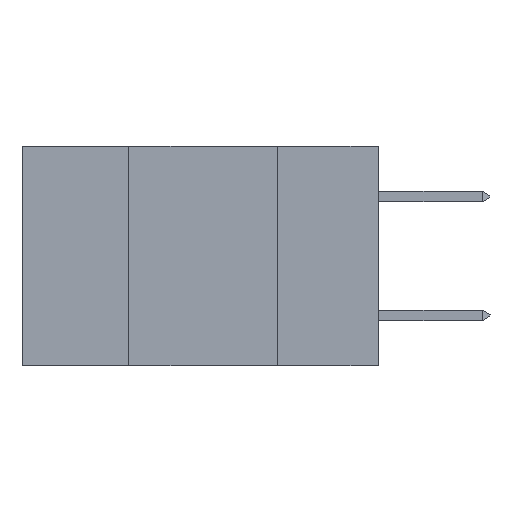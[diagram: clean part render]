
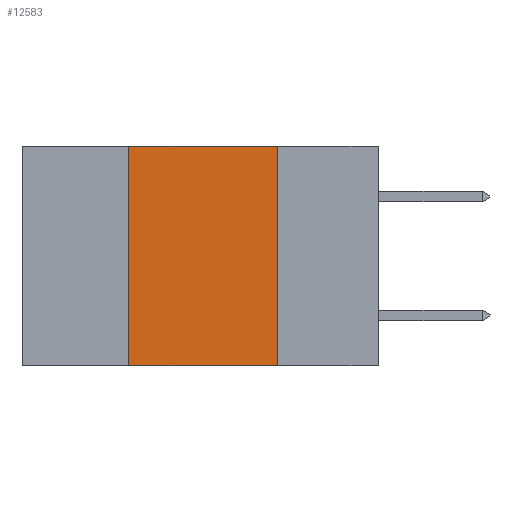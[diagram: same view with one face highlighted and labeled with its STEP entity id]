
A CAD part, left-side view. The second image highlights one B-rep face of the part: STEP entity #12583.
In plain terms, the highlighted planar face has unit normal (-1, 0, 0).
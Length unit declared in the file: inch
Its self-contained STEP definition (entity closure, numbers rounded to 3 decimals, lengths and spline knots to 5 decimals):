
#80 = CARTESIAN_POINT ( 'NONE',  ( 0., 0.17, 0. ) ) ;
#512 = VERTEX_POINT ( 'NONE', #23130 ) ;
#841 = DIRECTION ( 'NONE',  ( 0., 0., -1. ) ) ;
#984 = VECTOR ( 'NONE', #2946, 39.37008 ) ;
#2946 = DIRECTION ( 'NONE',  ( 0., 0., 1. ) ) ;
#3130 = CARTESIAN_POINT ( 'NONE',  ( 0., 0.17, 0. ) ) ;
#5630 = FACE_OUTER_BOUND ( 'NONE', #9702, .T. ) ;
#6082 = ORIENTED_EDGE ( 'NONE', *, *, #6655, .F. ) ;
#6303 = VERTEX_POINT ( 'NONE', #14088 ) ;
#6655 = EDGE_CURVE ( 'NONE', #512, #19366, #23656, .T. ) ;
#8643 = EDGE_CURVE ( 'NONE', #19366, #18771, #22500, .T. ) ;
#8821 = CARTESIAN_POINT ( 'NONE',  ( 0., 0.6, 0. ) ) ;
#9683 = CARTESIAN_POINT ( 'NONE',  ( 0., 0.6, 0. ) ) ;
#9702 = EDGE_LOOP ( 'NONE', ( #20387, #15675, #6082, #18639 ) ) ;
#10655 = CARTESIAN_POINT ( 'NONE',  ( 0., 0.6, -0.37 ) ) ;
#11892 = PLANE ( 'NONE',  #14890 ) ;
#12583 = ADVANCED_FACE ( 'NONE', ( #5630 ), #11892, .F. ) ;
#12701 = VECTOR ( 'NONE', #25864, 39.37008 ) ;
#12941 = VECTOR ( 'NONE', #13301, 39.37008 ) ;
#13301 = DIRECTION ( 'NONE',  ( 0., 0., -1. ) ) ;
#14056 = DIRECTION ( 'NONE',  ( 1., 0., 0. ) ) ;
#14088 = CARTESIAN_POINT ( 'NONE',  ( 0., 0.17, -0.37 ) ) ;
#14890 = AXIS2_PLACEMENT_3D ( 'NONE', #9683, #14056, #841 ) ;
#15675 = ORIENTED_EDGE ( 'NONE', *, *, #8643, .F. ) ;
#16690 = VECTOR ( 'NONE', #27375, 39.37008 ) ;
#18639 = ORIENTED_EDGE ( 'NONE', *, *, #20947, .T. ) ;
#18771 = VERTEX_POINT ( 'NONE', #3130 ) ;
#19366 = VERTEX_POINT ( 'NONE', #22595 ) ;
#20387 = ORIENTED_EDGE ( 'NONE', *, *, #22242, .F. ) ;
#20947 = EDGE_CURVE ( 'NONE', #512, #6303, #23611, .T. ) ;
#21543 = CARTESIAN_POINT ( 'NONE',  ( 0., 0.42, 0. ) ) ;
#22242 = EDGE_CURVE ( 'NONE', #18771, #6303, #25194, .T. ) ;
#22500 = LINE ( 'NONE', #8821, #16690 ) ;
#22595 = CARTESIAN_POINT ( 'NONE',  ( 0., 0.42, 0. ) ) ;
#23130 = CARTESIAN_POINT ( 'NONE',  ( 0., 0.42, -0.37 ) ) ;
#23611 = LINE ( 'NONE', #10655, #12701 ) ;
#23656 = LINE ( 'NONE', #21543, #984 ) ;
#25194 = LINE ( 'NONE', #80, #12941 ) ;
#25864 = DIRECTION ( 'NONE',  ( 0., -1., 0. ) ) ;
#27375 = DIRECTION ( 'NONE',  ( 0., -1., 0. ) ) ;
